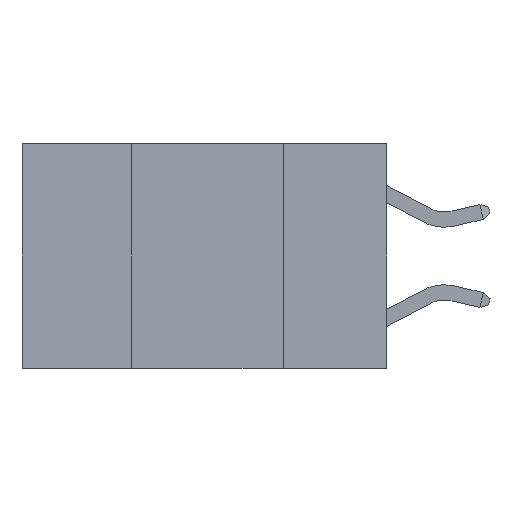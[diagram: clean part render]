
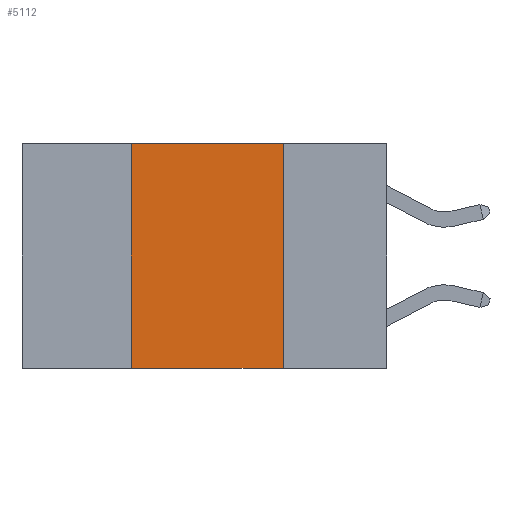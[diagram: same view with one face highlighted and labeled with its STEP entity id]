
A CAD part, left-side view. The second image highlights one B-rep face of the part: STEP entity #5112.
In plain terms, the highlighted planar face has unit normal (-1, 0, 0).
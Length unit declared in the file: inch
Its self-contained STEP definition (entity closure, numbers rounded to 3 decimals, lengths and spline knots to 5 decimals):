
#273 = CARTESIAN_POINT ( 'NONE',  ( 0., 0.17, 0. ) ) ;
#360 = CARTESIAN_POINT ( 'NONE',  ( 0., 0.42, -0.37 ) ) ;
#898 = LINE ( 'NONE', #24624, #22781 ) ;
#2157 = CARTESIAN_POINT ( 'NONE',  ( 0., 0.6, 0. ) ) ;
#2244 = EDGE_LOOP ( 'NONE', ( #3261, #14518, #26509, #10203 ) ) ;
#3261 = ORIENTED_EDGE ( 'NONE', *, *, #26654, .F. ) ;
#5112 = ADVANCED_FACE ( 'NONE', ( #23582 ), #8393, .F. ) ;
#6362 = DIRECTION ( 'NONE',  ( 1., 0., 0. ) ) ;
#7074 = LINE ( 'NONE', #12140, #23391 ) ;
#8393 = PLANE ( 'NONE',  #25214 ) ;
#8510 = VERTEX_POINT ( 'NONE', #8637 ) ;
#8637 = CARTESIAN_POINT ( 'NONE',  ( 0., 0.17, 0. ) ) ;
#8816 = LINE ( 'NONE', #273, #25128 ) ;
#9016 = EDGE_CURVE ( 'NONE', #17312, #22901, #7074, .T. ) ;
#9500 = CARTESIAN_POINT ( 'NONE',  ( 0., 0.42, 0. ) ) ;
#9600 = CARTESIAN_POINT ( 'NONE',  ( 0., 0.42, 0. ) ) ;
#9725 = DIRECTION ( 'NONE',  ( 0., -1., 0. ) ) ;
#10203 = ORIENTED_EDGE ( 'NONE', *, *, #9016, .T. ) ;
#11865 = EDGE_CURVE ( 'NONE', #17312, #16209, #11920, .T. ) ;
#11920 = LINE ( 'NONE', #9500, #17586 ) ;
#12140 = CARTESIAN_POINT ( 'NONE',  ( 0., 0.6, -0.37 ) ) ;
#12469 = CARTESIAN_POINT ( 'NONE',  ( 0., 0.17, -0.37 ) ) ;
#14463 = DIRECTION ( 'NONE',  ( 0., -1., 0. ) ) ;
#14518 = ORIENTED_EDGE ( 'NONE', *, *, #15089, .F. ) ;
#15089 = EDGE_CURVE ( 'NONE', #16209, #8510, #898, .T. ) ;
#16209 = VERTEX_POINT ( 'NONE', #9600 ) ;
#17312 = VERTEX_POINT ( 'NONE', #360 ) ;
#17586 = VECTOR ( 'NONE', #22253, 39.37008 ) ;
#21232 = DIRECTION ( 'NONE',  ( 0., 0., -1. ) ) ;
#22253 = DIRECTION ( 'NONE',  ( 0., 0., 1. ) ) ;
#22781 = VECTOR ( 'NONE', #9725, 39.37008 ) ;
#22901 = VERTEX_POINT ( 'NONE', #12469 ) ;
#23391 = VECTOR ( 'NONE', #14463, 39.37008 ) ;
#23536 = DIRECTION ( 'NONE',  ( 0., 0., -1. ) ) ;
#23582 = FACE_OUTER_BOUND ( 'NONE', #2244, .T. ) ;
#24624 = CARTESIAN_POINT ( 'NONE',  ( 0., 0.6, 0. ) ) ;
#25128 = VECTOR ( 'NONE', #23536, 39.37008 ) ;
#25214 = AXIS2_PLACEMENT_3D ( 'NONE', #2157, #6362, #21232 ) ;
#26509 = ORIENTED_EDGE ( 'NONE', *, *, #11865, .F. ) ;
#26654 = EDGE_CURVE ( 'NONE', #8510, #22901, #8816, .T. ) ;
